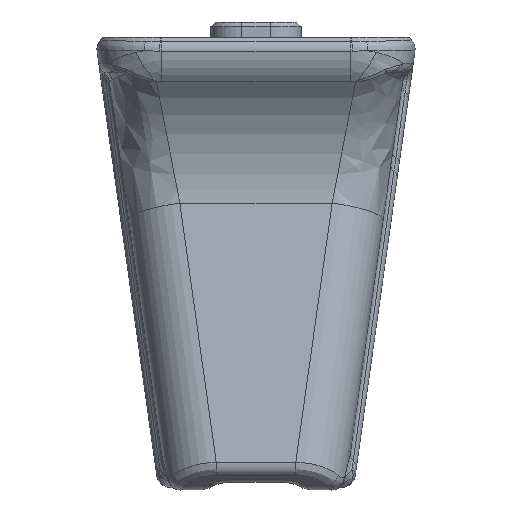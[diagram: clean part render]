
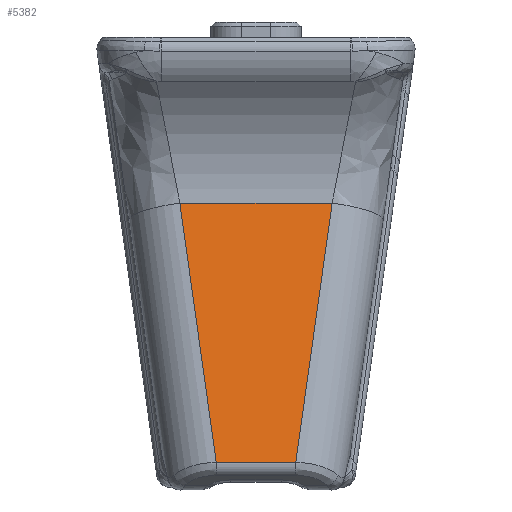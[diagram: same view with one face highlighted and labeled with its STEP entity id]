
A CAD part, front view. The second image highlights one B-rep face of the part: STEP entity #5382.
In plain terms, the highlighted planar face has unit normal (0, -0.984, 0.18).
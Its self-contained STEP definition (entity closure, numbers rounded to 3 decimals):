
#134=PLANE('',#5781);
#204=LINE('',#8555,#462);
#349=LINE('',#12074,#607);
#354=LINE('',#12160,#612);
#384=LINE('',#13793,#642);
#462=VECTOR('',#6027,10.);
#607=VECTOR('',#6560,10.);
#612=VECTOR('',#6597,10.);
#642=VECTOR('',#6787,10.);
#1053=FACE_OUTER_BOUND('',#1409,.T.);
#1409=EDGE_LOOP('',(#4769,#4770,#4771,#4772));
#2062=VERTEX_POINT('',#8470);
#2072=VERTEX_POINT('',#8554);
#2332=VERTEX_POINT('',#12070);
#2341=VERTEX_POINT('',#12158);
#2619=EDGE_CURVE('',#2072,#2062,#204,.T.);
#3049=EDGE_CURVE('',#2062,#2332,#349,.T.);
#3067=EDGE_CURVE('',#2341,#2332,#354,.T.);
#3206=EDGE_CURVE('',#2341,#2072,#384,.T.);
#4769=ORIENTED_EDGE('',*,*,#3049,.T.);
#4770=ORIENTED_EDGE('',*,*,#3067,.F.);
#4771=ORIENTED_EDGE('',*,*,#3206,.T.);
#4772=ORIENTED_EDGE('',*,*,#2619,.T.);
#5382=ADVANCED_FACE('',(#1053),#134,.F.);
#5781=AXIS2_PLACEMENT_3D('',#13792,#6785,#6786);
#6027=DIRECTION('',(0.137,-0.179,-0.974));
#6560=DIRECTION('',(1.,0.,0.));
#6597=DIRECTION('',(-0.137,-0.179,-0.974));
#6785=DIRECTION('center_axis',(0.,0.984,-0.18));
#6786=DIRECTION('ref_axis',(0.,-0.18,-0.984));
#6787=DIRECTION('',(-1.,0.,0.));
#8470=CARTESIAN_POINT('',(-3.086,-78.58,-35.805));
#8554=CARTESIAN_POINT('',(-5.916,-74.887,-15.672));
#8555=CARTESIAN_POINT('',(-5.872,-74.944,-15.983));
#12070=CARTESIAN_POINT('',(3.086,-78.58,-35.805));
#12074=CARTESIAN_POINT('',(-12.5,-78.58,-35.805));
#12158=CARTESIAN_POINT('',(5.916,-74.887,-15.672));
#12160=CARTESIAN_POINT('',(5.872,-74.944,-15.983));
#13792=CARTESIAN_POINT('Origin',(12.5,-74.887,-15.672));
#13793=CARTESIAN_POINT('',(12.5,-74.887,-15.672));
